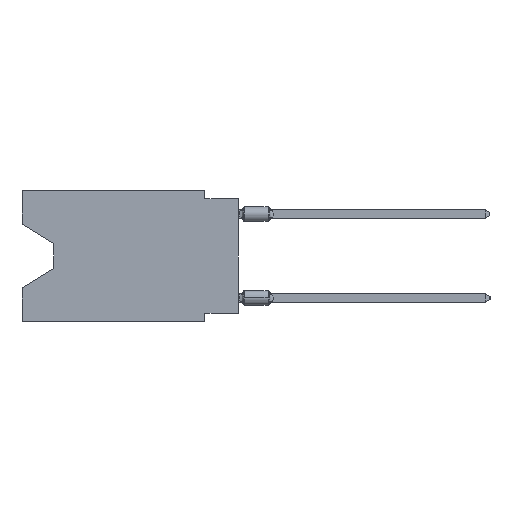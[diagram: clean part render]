
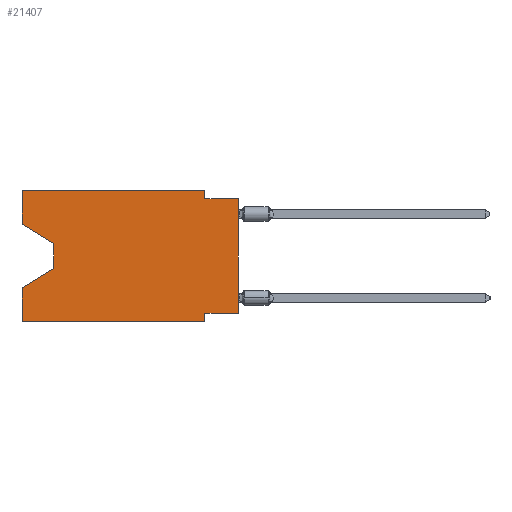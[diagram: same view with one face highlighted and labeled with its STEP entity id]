
A CAD part, left-side view. The second image highlights one B-rep face of the part: STEP entity #21407.
In plain terms, the highlighted planar face has unit normal (-1, 0, 0).
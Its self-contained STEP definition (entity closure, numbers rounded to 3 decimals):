
#2309 = EDGE_CURVE ( 'NONE', #10925, #20468, #2856, .T. ) ;
#2782 = VERTEX_POINT ( 'NONE', #41671 ) ;
#2856 = LINE ( 'NONE', #41049, #30148 ) ;
#3729 = LINE ( 'NONE', #28193, #20901 ) ;
#3822 = ORIENTED_EDGE ( 'NONE', *, *, #11134, .T. ) ;
#3900 = DIRECTION ( 'NONE',  ( 0., 0., 1. ) ) ;
#4007 = CARTESIAN_POINT ( 'NONE',  ( 0., 2.54, 0. ) ) ;
#4132 = LINE ( 'NONE', #28590, #24550 ) ;
#4219 = DIRECTION ( 'NONE',  ( 0., -0.855, -0.519 ) ) ;
#4374 = ORIENTED_EDGE ( 'NONE', *, *, #16738, .F. ) ;
#4844 = ORIENTED_EDGE ( 'NONE', *, *, #7981, .T. ) ;
#5132 = EDGE_CURVE ( 'NONE', #16346, #18292, #32744, .T. ) ;
#5225 = AXIS2_PLACEMENT_3D ( 'NONE', #42029, #29379, #38144 ) ;
#5807 = VERTEX_POINT ( 'NONE', #28430 ) ;
#6801 = PLANE ( 'NONE',  #5225 ) ;
#6804 = VERTEX_POINT ( 'NONE', #19403 ) ;
#7454 = CARTESIAN_POINT ( 'NONE',  ( 0., 16.383, -9.906 ) ) ;
#7981 = EDGE_CURVE ( 'NONE', #6804, #2782, #41119, .T. ) ;
#8080 = CARTESIAN_POINT ( 'NONE',  ( 0., 16.383, -7.36 ) ) ;
#8671 = EDGE_CURVE ( 'NONE', #5807, #10925, #42401, .T. ) ;
#9029 = LINE ( 'NONE', #39449, #25876 ) ;
#9688 = EDGE_CURVE ( 'NONE', #6804, #12724, #9029, .T. ) ;
#9737 = ORIENTED_EDGE ( 'NONE', *, *, #33954, .F. ) ;
#9940 = DIRECTION ( 'NONE',  ( 0., 0., -1. ) ) ;
#10925 = VERTEX_POINT ( 'NONE', #25546 ) ;
#11075 = CARTESIAN_POINT ( 'NONE',  ( 0., 16.383, -2.546 ) ) ;
#11134 = EDGE_CURVE ( 'NONE', #20468, #18292, #39176, .T. ) ;
#12724 = VERTEX_POINT ( 'NONE', #33528 ) ;
#13817 = EDGE_CURVE ( 'NONE', #12724, #40235, #41982, .T. ) ;
#14120 = FACE_OUTER_BOUND ( 'NONE', #35379, .T. ) ;
#14579 = LINE ( 'NONE', #35627, #29408 ) ;
#15725 = CARTESIAN_POINT ( 'NONE',  ( 0., 2.54, -0.635 ) ) ;
#16346 = VERTEX_POINT ( 'NONE', #7454 ) ;
#16622 = CARTESIAN_POINT ( 'NONE',  ( 0., 2.54, 0. ) ) ;
#16738 = EDGE_CURVE ( 'NONE', #43620, #43499, #35335, .T. ) ;
#17238 = ORIENTED_EDGE ( 'NONE', *, *, #33698, .F. ) ;
#17493 = VECTOR ( 'NONE', #43969, 1000. ) ;
#17507 = LINE ( 'NONE', #42213, #18237 ) ;
#17872 = ORIENTED_EDGE ( 'NONE', *, *, #8671, .T. ) ;
#18237 = VECTOR ( 'NONE', #24590, 1000. ) ;
#18292 = VERTEX_POINT ( 'NONE', #8080 ) ;
#19403 = CARTESIAN_POINT ( 'NONE',  ( 0., 0., -9.271 ) ) ;
#19799 = ORIENTED_EDGE ( 'NONE', *, *, #9688, .F. ) ;
#20468 = VERTEX_POINT ( 'NONE', #22141 ) ;
#20901 = VECTOR ( 'NONE', #38723, 1000. ) ;
#21407 = ADVANCED_FACE ( 'NONE', ( #14120 ), #6801, .F. ) ;
#22141 = CARTESIAN_POINT ( 'NONE',  ( 0., 13.97, -5.893 ) ) ;
#22786 = EDGE_CURVE ( 'NONE', #16346, #40235, #14579, .T. ) ;
#23098 = VECTOR ( 'NONE', #28413, 1000. ) ;
#24550 = VECTOR ( 'NONE', #3900, 1000. ) ;
#24590 = DIRECTION ( 'NONE',  ( 0., -1., 0. ) ) ;
#24930 = DIRECTION ( 'NONE',  ( 0., 0., 1. ) ) ;
#25301 = VERTEX_POINT ( 'NONE', #44846 ) ;
#25546 = CARTESIAN_POINT ( 'NONE',  ( 0., 13.97, -4.013 ) ) ;
#25876 = VECTOR ( 'NONE', #32592, 1000. ) ;
#27567 = VECTOR ( 'NONE', #43670, 1000. ) ;
#28021 = DIRECTION ( 'NONE',  ( 0., 0., -1. ) ) ;
#28193 = CARTESIAN_POINT ( 'NONE',  ( 0., 0., -0.635 ) ) ;
#28413 = DIRECTION ( 'NONE',  ( 0., 0.855, -0.519 ) ) ;
#28430 = CARTESIAN_POINT ( 'NONE',  ( 0., 16.383, -2.546 ) ) ;
#28523 = DIRECTION ( 'NONE',  ( 0., -1., 0. ) ) ;
#28590 = CARTESIAN_POINT ( 'NONE',  ( 0., 16.383, 0. ) ) ;
#29379 = DIRECTION ( 'NONE',  ( 1., 0., 0. ) ) ;
#29408 = VECTOR ( 'NONE', #28523, 1000. ) ;
#30148 = VECTOR ( 'NONE', #9940, 1000. ) ;
#31246 = CARTESIAN_POINT ( 'NONE',  ( 0., 2.54, -9.906 ) ) ;
#32592 = DIRECTION ( 'NONE',  ( 0., 1., 0. ) ) ;
#32744 = LINE ( 'NONE', #38903, #42831 ) ;
#33528 = CARTESIAN_POINT ( 'NONE',  ( 0., 2.54, -9.271 ) ) ;
#33698 = EDGE_CURVE ( 'NONE', #43499, #2782, #3729, .T. ) ;
#33954 = EDGE_CURVE ( 'NONE', #5807, #25301, #4132, .T. ) ;
#34297 = ORIENTED_EDGE ( 'NONE', *, *, #2309, .T. ) ;
#35059 = CARTESIAN_POINT ( 'NONE',  ( 0., 13.97, -5.893 ) ) ;
#35335 = LINE ( 'NONE', #4007, #17493 ) ;
#35379 = EDGE_LOOP ( 'NONE', ( #17872, #34297, #3822, #41684, #43096, #38146, #19799, #4844, #17238, #4374, #40337, #9737 ) ) ;
#35627 = CARTESIAN_POINT ( 'NONE',  ( 0., 16.383, -9.906 ) ) ;
#37024 = CARTESIAN_POINT ( 'NONE',  ( 0., 0., 0. ) ) ;
#38144 = DIRECTION ( 'NONE',  ( 0., 0., -1. ) ) ;
#38146 = ORIENTED_EDGE ( 'NONE', *, *, #13817, .F. ) ;
#38723 = DIRECTION ( 'NONE',  ( 0., -1., 0. ) ) ;
#38903 = CARTESIAN_POINT ( 'NONE',  ( 0., 16.383, 0. ) ) ;
#38963 = VECTOR ( 'NONE', #4219, 1000. ) ;
#39176 = LINE ( 'NONE', #35059, #23098 ) ;
#39449 = CARTESIAN_POINT ( 'NONE',  ( 0., 0., -9.271 ) ) ;
#40235 = VERTEX_POINT ( 'NONE', #44165 ) ;
#40337 = ORIENTED_EDGE ( 'NONE', *, *, #43733, .F. ) ;
#41049 = CARTESIAN_POINT ( 'NONE',  ( 0., 13.97, -4.013 ) ) ;
#41119 = LINE ( 'NONE', #37024, #27567 ) ;
#41671 = CARTESIAN_POINT ( 'NONE',  ( 0., 0., -0.635 ) ) ;
#41684 = ORIENTED_EDGE ( 'NONE', *, *, #5132, .F. ) ;
#41982 = LINE ( 'NONE', #31246, #42249 ) ;
#42029 = CARTESIAN_POINT ( 'NONE',  ( 0., 16.383, 0. ) ) ;
#42213 = CARTESIAN_POINT ( 'NONE',  ( 0., 16.383, 0. ) ) ;
#42249 = VECTOR ( 'NONE', #28021, 1000. ) ;
#42401 = LINE ( 'NONE', #11075, #38963 ) ;
#42831 = VECTOR ( 'NONE', #24930, 1000. ) ;
#43096 = ORIENTED_EDGE ( 'NONE', *, *, #22786, .T. ) ;
#43499 = VERTEX_POINT ( 'NONE', #15725 ) ;
#43620 = VERTEX_POINT ( 'NONE', #16622 ) ;
#43670 = DIRECTION ( 'NONE',  ( 0., 0., 1. ) ) ;
#43733 = EDGE_CURVE ( 'NONE', #25301, #43620, #17507, .T. ) ;
#43969 = DIRECTION ( 'NONE',  ( 0., 0., -1. ) ) ;
#44165 = CARTESIAN_POINT ( 'NONE',  ( 0., 2.54, -9.906 ) ) ;
#44846 = CARTESIAN_POINT ( 'NONE',  ( 0., 16.383, 0. ) ) ;
